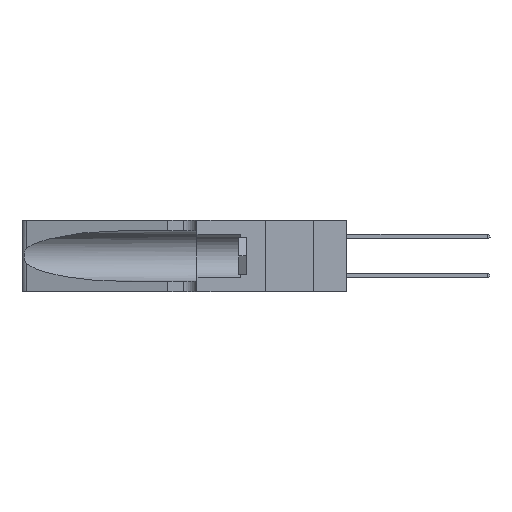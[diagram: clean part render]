
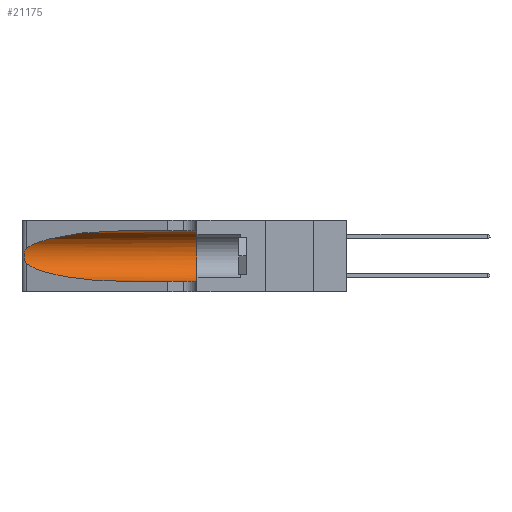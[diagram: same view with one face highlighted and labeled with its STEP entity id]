
A CAD part, left-side view. The second image highlights one B-rep face of the part: STEP entity #21175.
In plain terms, the highlighted cylindrical face has radius 3.308 mm (diameter 6.617 mm), a partial arc.
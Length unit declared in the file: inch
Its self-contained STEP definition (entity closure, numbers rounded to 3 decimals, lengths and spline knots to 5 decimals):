
#1150 = DIRECTION ( 'NONE',  ( 0., -1., 0. ) ) ;
#1203 = CARTESIAN_POINT ( 'NONE',  ( 0.25787, 1.23484, 0.2124 ) ) ;
#1581 = CARTESIAN_POINT ( 'NONE',  ( 0.1305, 0.35, 0.185 ) ) ;
#1717 =( BOUNDED_CURVE ( )  B_SPLINE_CURVE ( 3, ( #20906, #4630, #30723, #11253 ),
 .UNSPECIFIED., .F., .F. ) 
 B_SPLINE_CURVE_WITH_KNOTS ( ( 4, 4 ),
 ( 1.5708, 2.84003 ),
 .UNSPECIFIED. ) 
 CURVE ( )  GEOMETRIC_REPRESENTATION_ITEM ( )  RATIONAL_B_SPLINE_CURVE ( ( 1., 0.87, 0.87, 1. ) ) 
 REPRESENTATION_ITEM ( '' )  );
#2496 = VERTEX_POINT ( 'NONE', #29749 ) ;
#4301 = ORIENTED_EDGE ( 'NONE', *, *, #33766, .T. ) ;
#4536 = CARTESIAN_POINT ( 'NONE',  ( 0.26018, 1.23835, 0.19895 ) ) ;
#4630 = CARTESIAN_POINT ( 'NONE',  ( 0.18966, 0.96281, 0.31525 ) ) ;
#4897 = DIRECTION ( 'NONE',  ( 0., 0., 1. ) ) ;
#5532 = DIRECTION ( 'NONE',  ( 0., -1., 0. ) ) ;
#7372 = ORIENTED_EDGE ( 'NONE', *, *, #37639, .T. ) ;
#7671 = CARTESIAN_POINT ( 'NONE',  ( 0.25487, 1.22718, 0.22369 ) ) ;
#7816 = CARTESIAN_POINT ( 'NONE',  ( 0.26075, 1.23896, 0.178 ) ) ;
#8212 = CARTESIAN_POINT ( 'NONE',  ( 0.25487, 1.22718, 0.22369 ) ) ;
#9342 =( BOUNDED_CURVE ( )  B_SPLINE_CURVE ( 3, ( #32309, #29169, #12997, #35733 ),
 .UNSPECIFIED., .F., .F. ) 
 B_SPLINE_CURVE_WITH_KNOTS ( ( 4, 4 ),
 ( 3.44316, 4.71239 ),
 .UNSPECIFIED. ) 
 CURVE ( )  GEOMETRIC_REPRESENTATION_ITEM ( )  RATIONAL_B_SPLINE_CURVE ( ( 1., 0.87, 0.87, 1. ) ) 
 REPRESENTATION_ITEM ( '' )  );
#9429 = ORIENTED_EDGE ( 'NONE', *, *, #25177, .T. ) ;
#11146 = CARTESIAN_POINT ( 'NONE',  ( 0.25856, 1.23593, 0.16098 ) ) ;
#11253 = CARTESIAN_POINT ( 'NONE',  ( 0.25487, 1.22718, 0.22369 ) ) ;
#11438 = CARTESIAN_POINT ( 'NONE',  ( 0.1305, 1.61858, 0.185 ) ) ;
#11959 = VERTEX_POINT ( 'NONE', #32004 ) ;
#12916 = LINE ( 'NONE', #18552, #31206 ) ;
#12997 = CARTESIAN_POINT ( 'NONE',  ( 0.18966, 0.96281, 0.05475 ) ) ;
#13106 = CIRCLE ( 'NONE', #20512, 0.13025 ) ;
#14443 = CARTESIAN_POINT ( 'NONE',  ( 0.25639, 1.23186, 0.15144 ) ) ;
#14610 = ORIENTED_EDGE ( 'NONE', *, *, #31951, .F. ) ;
#14897 = CARTESIAN_POINT ( 'NONE',  ( 0.1305, 0.72297, 0.31525 ) ) ;
#16111 = ORIENTED_EDGE ( 'NONE', *, *, #33497, .T. ) ;
#16649 = CARTESIAN_POINT ( 'NONE',  ( 0.1305, 0.72297, 0.05475 ) ) ;
#17695 = CARTESIAN_POINT ( 'NONE',  ( 0.25487, 1.22718, 0.14631 ) ) ;
#18151 = ORIENTED_EDGE ( 'NONE', *, *, #29010, .F. ) ;
#18552 = CARTESIAN_POINT ( 'NONE',  ( 0.1305, 1.61858, 0.31525 ) ) ;
#18576 = CARTESIAN_POINT ( 'NONE',  ( 0.1305, 0.35, 0.05475 ) ) ;
#20512 = AXIS2_PLACEMENT_3D ( 'NONE', #1581, #24421, #4897 ) ;
#20812 = CARTESIAN_POINT ( 'NONE',  ( 0.25639, 1.23184, 0.21858 ) ) ;
#20906 = CARTESIAN_POINT ( 'NONE',  ( 0.1305, 0.72297, 0.31525 ) ) ;
#21175 = ADVANCED_FACE ( 'NONE', ( #33133 ), #23441, .F. ) ;
#21224 = DIRECTION ( 'NONE',  ( 0., 0., -1. ) ) ;
#23441 = CYLINDRICAL_SURFACE ( 'NONE', #32591, 0.13025 ) ;
#24065 = CARTESIAN_POINT ( 'NONE',  ( 0.25854, 1.2359, 0.20912 ) ) ;
#24421 = DIRECTION ( 'NONE',  ( 0., 1., 0. ) ) ;
#25177 = EDGE_CURVE ( 'NONE', #34107, #26125, #41434, .T. ) ;
#26125 = VERTEX_POINT ( 'NONE', #18576 ) ;
#27351 = CARTESIAN_POINT ( 'NONE',  ( 0.26075, 1.23896, 0.19203 ) ) ;
#29010 = EDGE_CURVE ( 'NONE', #2496, #26125, #13106, .T. ) ;
#29169 = CARTESIAN_POINT ( 'NONE',  ( 0.2373, 1.15595, 0.08982 ) ) ;
#29749 = CARTESIAN_POINT ( 'NONE',  ( 0.1305, 0.35, 0.31525 ) ) ;
#30424 = CARTESIAN_POINT ( 'NONE',  ( 0.1305, 1.61858, 0.05475 ) ) ;
#30616 = CARTESIAN_POINT ( 'NONE',  ( 0.26017, 1.23833, 0.17102 ) ) ;
#30723 = CARTESIAN_POINT ( 'NONE',  ( 0.2373, 1.15595, 0.28018 ) ) ;
#31206 = VECTOR ( 'NONE', #5532, 39.37008 ) ;
#31951 = EDGE_CURVE ( 'NONE', #39284, #2496, #12916, .T. ) ;
#32004 = CARTESIAN_POINT ( 'NONE',  ( 0.25487, 1.22718, 0.14631 ) ) ;
#32309 = CARTESIAN_POINT ( 'NONE',  ( 0.25487, 1.22718, 0.14631 ) ) ;
#32405 = VERTEX_POINT ( 'NONE', #8212 ) ;
#32591 = AXIS2_PLACEMENT_3D ( 'NONE', #11438, #40724, #21224 ) ;
#32772 = VECTOR ( 'NONE', #1150, 39.37008 ) ;
#33133 = FACE_OUTER_BOUND ( 'NONE', #41721, .T. ) ;
#33497 = EDGE_CURVE ( 'NONE', #11959, #34107, #9342, .T. ) ;
#33763 = CARTESIAN_POINT ( 'NONE',  ( 0.25555, 1.22994, 0.2215 ) ) ;
#33766 = EDGE_CURVE ( 'NONE', #39284, #32405, #1717, .T. ) ;
#33903 = CARTESIAN_POINT ( 'NONE',  ( 0.25789, 1.23486, 0.15765 ) ) ;
#34107 = VERTEX_POINT ( 'NONE', #16649 ) ;
#35733 = CARTESIAN_POINT ( 'NONE',  ( 0.1305, 0.72297, 0.05475 ) ) ;
#36518 = B_SPLINE_CURVE_WITH_KNOTS ( 'NONE', 3,
 ( #7671, #33763, #20812, #1203, #24065, #4536, #27351, #7816, #30616, #11146, #33903, #14443, #37187, #17695 ),
 .UNSPECIFIED., .F., .F.,
 ( 4, 2, 2, 2, 2, 2, 4 ),
 ( 0., 0.00027, 0.00053, 0.00107, 0.0016, 0.00187, 0.00214 ),
 .UNSPECIFIED. ) ;
#37187 = CARTESIAN_POINT ( 'NONE',  ( 0.25555, 1.22993, 0.14849 ) ) ;
#37639 = EDGE_CURVE ( 'NONE', #32405, #11959, #36518, .T. ) ;
#39284 = VERTEX_POINT ( 'NONE', #14897 ) ;
#40724 = DIRECTION ( 'NONE',  ( 0., -1., 0. ) ) ;
#41434 = LINE ( 'NONE', #30424, #32772 ) ;
#41721 = EDGE_LOOP ( 'NONE', ( #4301, #7372, #16111, #9429, #18151, #14610 ) ) ;
